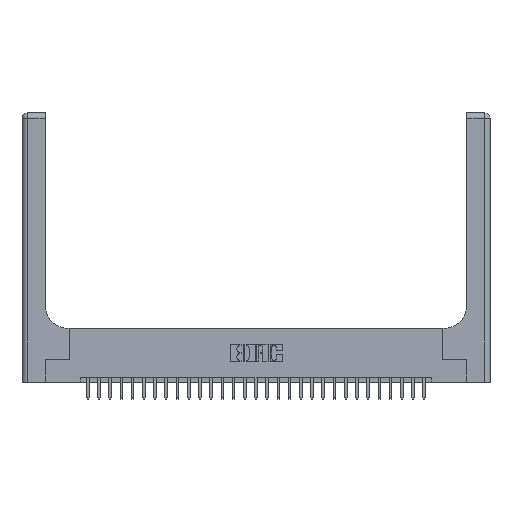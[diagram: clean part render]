
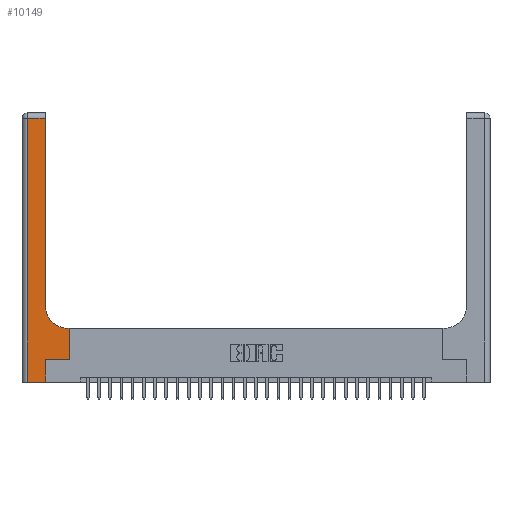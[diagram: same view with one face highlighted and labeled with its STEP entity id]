
A CAD part, top view. The second image highlights one B-rep face of the part: STEP entity #10149.
In plain terms, the highlighted planar face has unit normal (0, 0, 1).
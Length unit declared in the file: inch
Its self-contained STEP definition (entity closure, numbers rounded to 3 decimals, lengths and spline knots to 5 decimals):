
#27 = CIRCLE ( 'NONE', #26235, 0.25 ) ;
#80 = DIRECTION ( 'NONE',  ( -1., 0., 0. ) ) ;
#264 = DIRECTION ( 'NONE',  ( 1., 0., 0. ) ) ;
#629 = LINE ( 'NONE', #19103, #23976 ) ;
#813 = CARTESIAN_POINT ( 'NONE',  ( 0.06, 2.94, 0.37 ) ) ;
#860 = VECTOR ( 'NONE', #11492, 39.37008 ) ;
#1935 = LINE ( 'NONE', #14992, #7902 ) ;
#2092 = DIRECTION ( 'NONE',  ( 0., 1., 0. ) ) ;
#2301 = VERTEX_POINT ( 'NONE', #25260 ) ;
#2919 = DIRECTION ( 'NONE',  ( -1., 0., 0. ) ) ;
#3082 = CARTESIAN_POINT ( 'NONE',  ( 0.265, 0., 0.37 ) ) ;
#3480 = VECTOR ( 'NONE', #21350, 39.37008 ) ;
#3807 = DIRECTION ( 'NONE',  ( 1., 0., 0. ) ) ;
#4062 = VECTOR ( 'NONE', #3807, 39.37008 ) ;
#4644 = VERTEX_POINT ( 'NONE', #15867 ) ;
#4840 = ORIENTED_EDGE ( 'NONE', *, *, #5033, .T. ) ;
#4980 = CARTESIAN_POINT ( 'NONE',  ( 0.26, 0.85, 0.37 ) ) ;
#5033 = EDGE_CURVE ( 'NONE', #7409, #6384, #12671, .T. ) ;
#5093 = CARTESIAN_POINT ( 'NONE',  ( 0.06, 3., 0.37 ) ) ;
#5778 = ORIENTED_EDGE ( 'NONE', *, *, #14845, .T. ) ;
#5903 = ORIENTED_EDGE ( 'NONE', *, *, #23025, .T. ) ;
#6037 = CARTESIAN_POINT ( 'NONE',  ( 0., 0., 0.37 ) ) ;
#6318 = LINE ( 'NONE', #6037, #4062 ) ;
#6384 = VERTEX_POINT ( 'NONE', #23921 ) ;
#6472 = CARTESIAN_POINT ( 'NONE',  ( 0.265, 0., 0.37 ) ) ;
#7409 = VERTEX_POINT ( 'NONE', #4980 ) ;
#7902 = VECTOR ( 'NONE', #264, 39.37008 ) ;
#8164 = EDGE_CURVE ( 'NONE', #17305, #8451, #6318, .T. ) ;
#8451 = VERTEX_POINT ( 'NONE', #3082 ) ;
#10149 = ADVANCED_FACE ( 'NONE', ( #21975 ), #26549, .F. ) ;
#10584 = VERTEX_POINT ( 'NONE', #813 ) ;
#10612 = DIRECTION ( 'NONE',  ( 0., 1., 0. ) ) ;
#10713 = CARTESIAN_POINT ( 'NONE',  ( 0.51, 0.85, 0.37 ) ) ;
#11492 = DIRECTION ( 'NONE',  ( 0., -1., 0. ) ) ;
#11591 = EDGE_CURVE ( 'NONE', #2301, #4644, #1935, .T. ) ;
#11933 = CARTESIAN_POINT ( 'NONE',  ( 0.06, 0., 0.37 ) ) ;
#12319 = LINE ( 'NONE', #6472, #3480 ) ;
#12671 = LINE ( 'NONE', #21137, #22194 ) ;
#12702 = VERTEX_POINT ( 'NONE', #17288 ) ;
#12960 = ORIENTED_EDGE ( 'NONE', *, *, #19244, .T. ) ;
#13523 = EDGE_CURVE ( 'NONE', #10584, #17305, #25959, .T. ) ;
#13807 = CARTESIAN_POINT ( 'NONE',  ( 0.26, 0.6, 0.37 ) ) ;
#13894 = ORIENTED_EDGE ( 'NONE', *, *, #8164, .T. ) ;
#14035 = CARTESIAN_POINT ( 'NONE',  ( 0., 3., 0.37 ) ) ;
#14213 = ORIENTED_EDGE ( 'NONE', *, *, #11591, .T. ) ;
#14508 = AXIS2_PLACEMENT_3D ( 'NONE', #14035, #22383, #2919 ) ;
#14845 = EDGE_CURVE ( 'NONE', #12702, #7409, #27, .T. ) ;
#14992 = CARTESIAN_POINT ( 'NONE',  ( 0.265, 0.25, 0.37 ) ) ;
#15097 = VECTOR ( 'NONE', #10612, 39.37008 ) ;
#15297 = ORIENTED_EDGE ( 'NONE', *, *, #23347, .T. ) ;
#15867 = CARTESIAN_POINT ( 'NONE',  ( 0.528, 0.25, 0.37 ) ) ;
#16259 = VERTEX_POINT ( 'NONE', #24524 ) ;
#16545 = DIRECTION ( 'NONE',  ( 1., 0., 0. ) ) ;
#16643 = LINE ( 'NONE', #13807, #24894 ) ;
#17288 = CARTESIAN_POINT ( 'NONE',  ( 0.51, 0.6, 0.37 ) ) ;
#17305 = VERTEX_POINT ( 'NONE', #11933 ) ;
#18927 = CARTESIAN_POINT ( 'NONE',  ( 0.528, 0.25, 0.37 ) ) ;
#19085 = EDGE_LOOP ( 'NONE', ( #4840, #27233, #20459, #13894, #12960, #14213, #5903, #15297, #5778 ) ) ;
#19103 = CARTESIAN_POINT ( 'NONE',  ( 0., 2.94, 0.37 ) ) ;
#19244 = EDGE_CURVE ( 'NONE', #8451, #2301, #12319, .T. ) ;
#20459 = ORIENTED_EDGE ( 'NONE', *, *, #13523, .T. ) ;
#21137 = CARTESIAN_POINT ( 'NONE',  ( 0.26, 3., 0.37 ) ) ;
#21308 = LINE ( 'NONE', #18927, #15097 ) ;
#21350 = DIRECTION ( 'NONE',  ( 0., 1., 0. ) ) ;
#21975 = FACE_OUTER_BOUND ( 'NONE', #19085, .T. ) ;
#22194 = VECTOR ( 'NONE', #2092, 39.37008 ) ;
#22383 = DIRECTION ( 'NONE',  ( 0., 0., -1. ) ) ;
#22740 = EDGE_CURVE ( 'NONE', #6384, #10584, #629, .T. ) ;
#23025 = EDGE_CURVE ( 'NONE', #4644, #16259, #21308, .T. ) ;
#23346 = DIRECTION ( 'NONE',  ( 0., 0., -1. ) ) ;
#23347 = EDGE_CURVE ( 'NONE', #16259, #12702, #16643, .T. ) ;
#23921 = CARTESIAN_POINT ( 'NONE',  ( 0.26, 2.94, 0.37 ) ) ;
#23976 = VECTOR ( 'NONE', #80, 39.37008 ) ;
#24524 = CARTESIAN_POINT ( 'NONE',  ( 0.528, 0.6, 0.37 ) ) ;
#24894 = VECTOR ( 'NONE', #25141, 39.37008 ) ;
#25141 = DIRECTION ( 'NONE',  ( -1., 0., 0. ) ) ;
#25260 = CARTESIAN_POINT ( 'NONE',  ( 0.265, 0.25, 0.37 ) ) ;
#25959 = LINE ( 'NONE', #5093, #860 ) ;
#26235 = AXIS2_PLACEMENT_3D ( 'NONE', #10713, #23346, #16545 ) ;
#26549 = PLANE ( 'NONE',  #14508 ) ;
#27233 = ORIENTED_EDGE ( 'NONE', *, *, #22740, .T. ) ;
